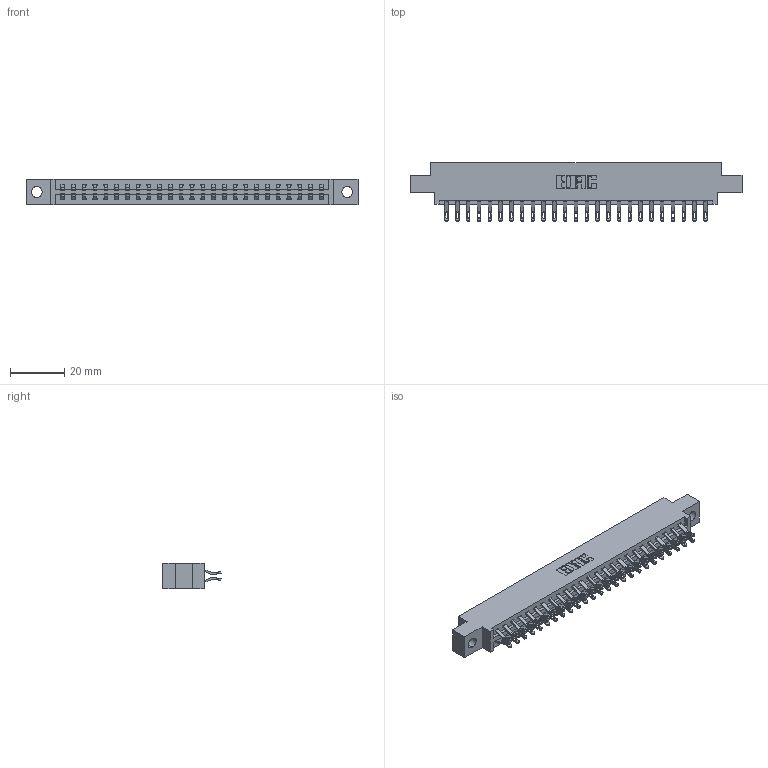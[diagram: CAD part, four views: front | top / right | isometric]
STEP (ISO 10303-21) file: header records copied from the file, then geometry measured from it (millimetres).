
FILE_DESCRIPTION (( 'STEP AP203' ), '1' );
FILE_NAME ('387-050-555-804.STEP', '2019-10-19T02:14:31', ( '' ), ( '' ), 'SwSTEP 2.0', 'SolidWorks 2016', '' );
FILE_SCHEMA (( 'CONFIG_CONTROL_DESIGN' ));
Length unit declared in the file: inch
Products named in the file (3): 337 Part_0.170 Offset - 0.156 Dia-TH; 345-292-001_555 Tail; 387-050-555-804
Assembly tree (51 placements, depth 2):
  387-050-555-804
    337 Part_0.170 Offset - 0.156 Dia-TH
    345-292-001_555 Tail  x50
Bounding box: 122.07 x 21.47 x 9.4 mm (x, y, z)
Volume: 12578.3 mm3; surface area: 14506.5 mm2
Topology: 51 solids, 51 shells, 3118 faces, 9773 edges, 6514 vertices
Faces by surface type: plane 1874, cylinder 1244
Entity records: 22043 total; most frequent: CARTESIAN_POINT 3764, ORIENTED_EDGE 3670, DIRECTION 3203, EDGE_CURVE 1835, VECTOR 1687, LINE 1687, VERTEX_POINT 1222, AXIS2_PLACEMENT_3D 758
